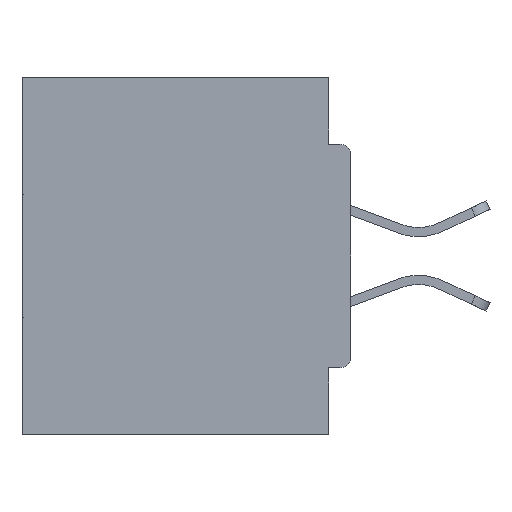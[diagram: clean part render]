
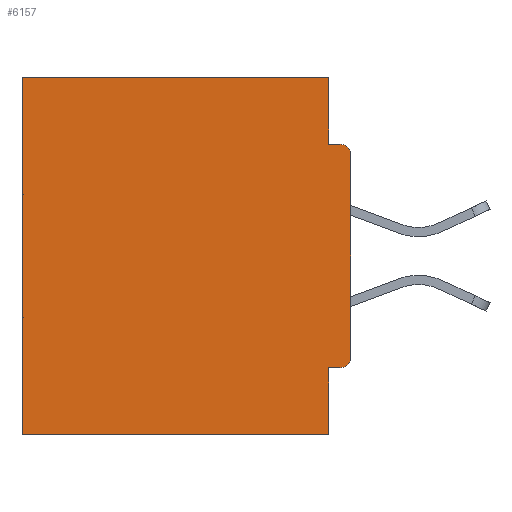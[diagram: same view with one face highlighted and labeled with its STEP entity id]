
A CAD part, left-side view. The second image highlights one B-rep face of the part: STEP entity #6157.
In plain terms, the highlighted planar face has unit normal (-1, 0, 0).
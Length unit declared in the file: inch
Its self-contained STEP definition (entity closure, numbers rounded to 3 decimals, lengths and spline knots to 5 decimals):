
#175 = FACE_OUTER_BOUND ( 'NONE', #38250, .T. ) ;
#347 = CARTESIAN_POINT ( 'NONE',  ( 0.298, 0.015, -0.1085 ) ) ;
#412 = PLANE ( 'NONE',  #26506 ) ;
#477 = VECTOR ( 'NONE', #11456, 39.37008 ) ;
#922 = VERTEX_POINT ( 'NONE', #25286 ) ;
#2110 = VECTOR ( 'NONE', #26278, 39.37008 ) ;
#2536 = ORIENTED_EDGE ( 'NONE', *, *, #21368, .F. ) ;
#2689 = EDGE_CURVE ( 'NONE', #19872, #31563, #18034, .T. ) ;
#3291 = VERTEX_POINT ( 'NONE', #37400 ) ;
#3329 = ORIENTED_EDGE ( 'NONE', *, *, #7716, .F. ) ;
#4916 = ORIENTED_EDGE ( 'NONE', *, *, #14496, .T. ) ;
#5415 = DIRECTION ( 'NONE',  ( 0., -1., 0. ) ) ;
#5976 = CARTESIAN_POINT ( 'NONE',  ( 0.298, 0., -0.0935 ) ) ;
#6157 = ADVANCED_FACE ( 'NONE', ( #175 ), #412, .F. ) ;
#6962 = DIRECTION ( 'NONE',  ( 0., 0., -1. ) ) ;
#7153 = CARTESIAN_POINT ( 'NONE',  ( 0.298, 0., 0. ) ) ;
#7413 = VERTEX_POINT ( 'NONE', #12644 ) ;
#7716 = EDGE_CURVE ( 'NONE', #10630, #31563, #16494, .T. ) ;
#8870 = LINE ( 'NONE', #39306, #2110 ) ;
#9088 = CARTESIAN_POINT ( 'NONE',  ( 0.298, 0., 0. ) ) ;
#9230 = DIRECTION ( 'NONE',  ( -1., 0., 0. ) ) ;
#9529 = ORIENTED_EDGE ( 'NONE', *, *, #12050, .F. ) ;
#9843 = VECTOR ( 'NONE', #40487, 39.37008 ) ;
#9845 = CIRCLE ( 'NONE', #15741, 0.015 ) ;
#10630 = VERTEX_POINT ( 'NONE', #29879 ) ;
#11456 = DIRECTION ( 'NONE',  ( 0., 1., 0. ) ) ;
#12050 = EDGE_CURVE ( 'NONE', #30671, #7413, #29415, .T. ) ;
#12124 = DIRECTION ( 'NONE',  ( 0., 0., -1. ) ) ;
#12644 = CARTESIAN_POINT ( 'NONE',  ( 0.298, 0.031, -0.0935 ) ) ;
#12804 = LINE ( 'NONE', #31134, #477 ) ;
#13248 = EDGE_CURVE ( 'NONE', #10630, #25088, #9845, .T. ) ;
#13724 = DIRECTION ( 'NONE',  ( -1., 0., 0. ) ) ;
#14496 = EDGE_CURVE ( 'NONE', #30671, #922, #20227, .T. ) ;
#15622 = LINE ( 'NONE', #16938, #18185 ) ;
#15741 = AXIS2_PLACEMENT_3D ( 'NONE', #347, #13724, #39788 ) ;
#16360 = ORIENTED_EDGE ( 'NONE', *, *, #33064, .F. ) ;
#16494 = LINE ( 'NONE', #9088, #30869 ) ;
#16544 = CARTESIAN_POINT ( 'NONE',  ( 0.298, 0.031, -0.5 ) ) ;
#16938 = CARTESIAN_POINT ( 'NONE',  ( 0.298, 0.031, -0.5 ) ) ;
#17131 = AXIS2_PLACEMENT_3D ( 'NONE', #28919, #9230, #32216 ) ;
#18034 = CIRCLE ( 'NONE', #17131, 0.015 ) ;
#18185 = VECTOR ( 'NONE', #6962, 39.37008 ) ;
#18662 = VECTOR ( 'NONE', #29722, 39.37008 ) ;
#19872 = VERTEX_POINT ( 'NONE', #31308 ) ;
#20227 = LINE ( 'NONE', #40764, #9843 ) ;
#20937 = VERTEX_POINT ( 'NONE', #16544 ) ;
#21272 = ORIENTED_EDGE ( 'NONE', *, *, #34075, .F. ) ;
#21309 = ORIENTED_EDGE ( 'NONE', *, *, #30886, .T. ) ;
#21368 = EDGE_CURVE ( 'NONE', #3291, #20937, #15622, .T. ) ;
#23041 = CARTESIAN_POINT ( 'NONE',  ( 0.298, 0., -0.4065 ) ) ;
#24139 = LINE ( 'NONE', #5976, #40973 ) ;
#24281 = CARTESIAN_POINT ( 'NONE',  ( 0.298, 0., -0.3915 ) ) ;
#25088 = VERTEX_POINT ( 'NONE', #30281 ) ;
#25286 = CARTESIAN_POINT ( 'NONE',  ( 0.298, 0.46, 0. ) ) ;
#26278 = DIRECTION ( 'NONE',  ( 0., 0., -1. ) ) ;
#26506 = AXIS2_PLACEMENT_3D ( 'NONE', #7153, #29715, #36723 ) ;
#28690 = LINE ( 'NONE', #23041, #36892 ) ;
#28919 = CARTESIAN_POINT ( 'NONE',  ( 0.298, 0.015, -0.3915 ) ) ;
#29415 = LINE ( 'NONE', #32748, #18662 ) ;
#29455 = ORIENTED_EDGE ( 'NONE', *, *, #2689, .T. ) ;
#29715 = DIRECTION ( 'NONE',  ( 1., 0., 0. ) ) ;
#29722 = DIRECTION ( 'NONE',  ( 0., 0., -1. ) ) ;
#29879 = CARTESIAN_POINT ( 'NONE',  ( 0.298, 0., -0.1085 ) ) ;
#30281 = CARTESIAN_POINT ( 'NONE',  ( 0.298, 0.015, -0.0935 ) ) ;
#30671 = VERTEX_POINT ( 'NONE', #35208 ) ;
#30869 = VECTOR ( 'NONE', #12124, 39.37008 ) ;
#30875 = CARTESIAN_POINT ( 'NONE',  ( 0.298, 0.46, -0.5 ) ) ;
#30886 = EDGE_CURVE ( 'NONE', #922, #40407, #8870, .T. ) ;
#31134 = CARTESIAN_POINT ( 'NONE',  ( 0.298, 0., -0.5 ) ) ;
#31308 = CARTESIAN_POINT ( 'NONE',  ( 0.298, 0.015, -0.4065 ) ) ;
#31563 = VERTEX_POINT ( 'NONE', #24281 ) ;
#32216 = DIRECTION ( 'NONE',  ( 0., 0., -1. ) ) ;
#32748 = CARTESIAN_POINT ( 'NONE',  ( 0.298, 0.031, -0.5 ) ) ;
#33064 = EDGE_CURVE ( 'NONE', #7413, #25088, #24139, .T. ) ;
#34075 = EDGE_CURVE ( 'NONE', #20937, #40407, #12804, .T. ) ;
#35208 = CARTESIAN_POINT ( 'NONE',  ( 0.298, 0.031, 0. ) ) ;
#35748 = DIRECTION ( 'NONE',  ( 0., 1., 0. ) ) ;
#36723 = DIRECTION ( 'NONE',  ( 0., 0., -1. ) ) ;
#36892 = VECTOR ( 'NONE', #35748, 39.37008 ) ;
#37400 = CARTESIAN_POINT ( 'NONE',  ( 0.298, 0.031, -0.4065 ) ) ;
#38250 = EDGE_LOOP ( 'NONE', ( #39873, #16360, #9529, #4916, #21309, #21272, #2536, #38851, #29455, #3329 ) ) ;
#38851 = ORIENTED_EDGE ( 'NONE', *, *, #42119, .F. ) ;
#39306 = CARTESIAN_POINT ( 'NONE',  ( 0.298, 0.46, 0. ) ) ;
#39788 = DIRECTION ( 'NONE',  ( 0., 0., -1. ) ) ;
#39873 = ORIENTED_EDGE ( 'NONE', *, *, #13248, .T. ) ;
#40407 = VERTEX_POINT ( 'NONE', #30875 ) ;
#40487 = DIRECTION ( 'NONE',  ( 0., 1., 0. ) ) ;
#40764 = CARTESIAN_POINT ( 'NONE',  ( 0.298, 0., 0. ) ) ;
#40973 = VECTOR ( 'NONE', #5415, 39.37008 ) ;
#42119 = EDGE_CURVE ( 'NONE', #19872, #3291, #28690, .T. ) ;
